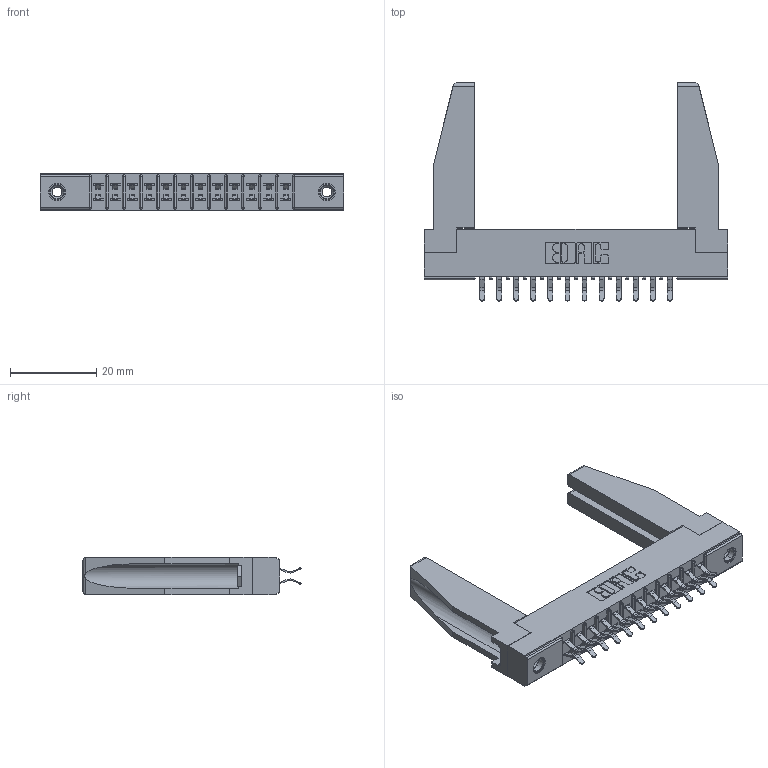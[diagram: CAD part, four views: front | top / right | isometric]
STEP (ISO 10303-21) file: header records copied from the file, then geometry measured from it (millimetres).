
FILE_DESCRIPTION (( 'STEP AP203' ), '1' );
FILE_NAME ('315-024-556-278.STEP', '2019-09-10T14:47:49', ( '' ), ( '' ), 'SwSTEP 2.0', 'SolidWorks 2016', '' );
FILE_SCHEMA (( 'CONFIG_CONTROL_DESIGN' ));
Length unit declared in the file: inch
Products named in the file (5): 315-024-556-278; 307-220-078; 305-290-001_556; 305 Part_.156 Dia; 345-250-001_345-250-001-102
Assembly tree (29 placements, depth 2):
  315-024-556-278
    305 Part_.156 Dia
    305-290-001_556  x24
    345-250-001_345-250-001-102  x2
    307-220-078  x2
Bounding box: 70.56 x 50.67 x 8.71 mm (x, y, z)
Volume: 8434.3 mm3; surface area: 11620.2 mm2
Topology: 29 solids, 29 shells, 1590 faces, 4522 edges, 2940 vertices
Faces by surface type: plane 896, cylinder 630, sphere 48, cone 12, torus 4
Entity records: 19306 total; most frequent: CARTESIAN_POINT 3204, ORIENTED_EDGE 3134, DIRECTION 3085, EDGE_CURVE 1567, VECTOR 1227, LINE 1227, VERTEX_POINT 1006, AXIS2_PLACEMENT_3D 929
